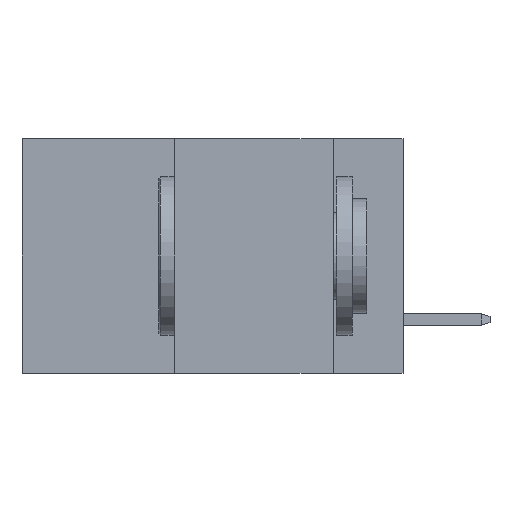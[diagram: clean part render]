
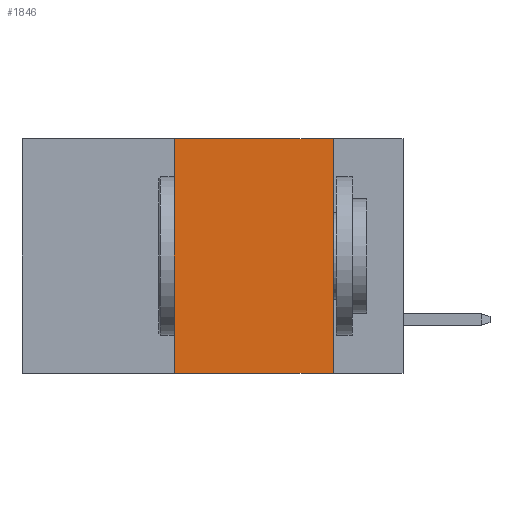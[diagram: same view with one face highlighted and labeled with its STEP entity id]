
A CAD part, left-side view. The second image highlights one B-rep face of the part: STEP entity #1846.
In plain terms, the highlighted planar face has unit normal (-1, 0, 0).
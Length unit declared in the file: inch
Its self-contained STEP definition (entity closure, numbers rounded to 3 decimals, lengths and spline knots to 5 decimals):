
#21 = PLANE ( 'NONE',  #8540 ) ;
#184 = EDGE_CURVE ( 'NONE', #8570, #7959, #7194, .T. ) ;
#1356 = LINE ( 'NONE', #4526, #1499 ) ;
#1499 = VECTOR ( 'NONE', #3993, 39.37008 ) ;
#1684 = EDGE_CURVE ( 'NONE', #8570, #4095, #5116, .T. ) ;
#1846 = ADVANCED_FACE ( 'NONE', ( #6242 ), #21, .F. ) ;
#1883 = CARTESIAN_POINT ( 'NONE',  ( 0., 0.11, -0.37 ) ) ;
#1973 = DIRECTION ( 'NONE',  ( 0., 0., 1. ) ) ;
#2368 = ORIENTED_EDGE ( 'NONE', *, *, #184, .T. ) ;
#2500 = DIRECTION ( 'NONE',  ( 0., 0., -1. ) ) ;
#2897 = EDGE_CURVE ( 'NONE', #6779, #7959, #4316, .T. ) ;
#2955 = ORIENTED_EDGE ( 'NONE', *, *, #1684, .F. ) ;
#3173 = CARTESIAN_POINT ( 'NONE',  ( 0., 0.6, 0. ) ) ;
#3301 = CARTESIAN_POINT ( 'NONE',  ( 0., 0.36, 0. ) ) ;
#3643 = CARTESIAN_POINT ( 'NONE',  ( 0., 0.6, -0.37 ) ) ;
#3993 = DIRECTION ( 'NONE',  ( 0., -1., 0. ) ) ;
#4095 = VERTEX_POINT ( 'NONE', #3301 ) ;
#4316 = LINE ( 'NONE', #5099, #10198 ) ;
#4468 = DIRECTION ( 'NONE',  ( 0., -1., 0. ) ) ;
#4526 = CARTESIAN_POINT ( 'NONE',  ( 0., 0.6, 0. ) ) ;
#4671 = DIRECTION ( 'NONE',  ( 1., 0., 0. ) ) ;
#4746 = VECTOR ( 'NONE', #4468, 39.37008 ) ;
#5099 = CARTESIAN_POINT ( 'NONE',  ( 0., 0.11, 0. ) ) ;
#5116 = LINE ( 'NONE', #9111, #6038 ) ;
#5514 = DIRECTION ( 'NONE',  ( 0., 0., -1. ) ) ;
#6038 = VECTOR ( 'NONE', #1973, 39.37008 ) ;
#6242 = FACE_OUTER_BOUND ( 'NONE', #8246, .T. ) ;
#6637 = ORIENTED_EDGE ( 'NONE', *, *, #9631, .F. ) ;
#6779 = VERTEX_POINT ( 'NONE', #7626 ) ;
#7194 = LINE ( 'NONE', #3643, #4746 ) ;
#7626 = CARTESIAN_POINT ( 'NONE',  ( 0., 0.11, 0. ) ) ;
#7959 = VERTEX_POINT ( 'NONE', #1883 ) ;
#8246 = EDGE_LOOP ( 'NONE', ( #8851, #6637, #2955, #2368 ) ) ;
#8540 = AXIS2_PLACEMENT_3D ( 'NONE', #3173, #4671, #5514 ) ;
#8570 = VERTEX_POINT ( 'NONE', #9747 ) ;
#8851 = ORIENTED_EDGE ( 'NONE', *, *, #2897, .F. ) ;
#9111 = CARTESIAN_POINT ( 'NONE',  ( 0., 0.36, 0. ) ) ;
#9631 = EDGE_CURVE ( 'NONE', #4095, #6779, #1356, .T. ) ;
#9747 = CARTESIAN_POINT ( 'NONE',  ( 0., 0.36, -0.37 ) ) ;
#10198 = VECTOR ( 'NONE', #2500, 39.37008 ) ;
